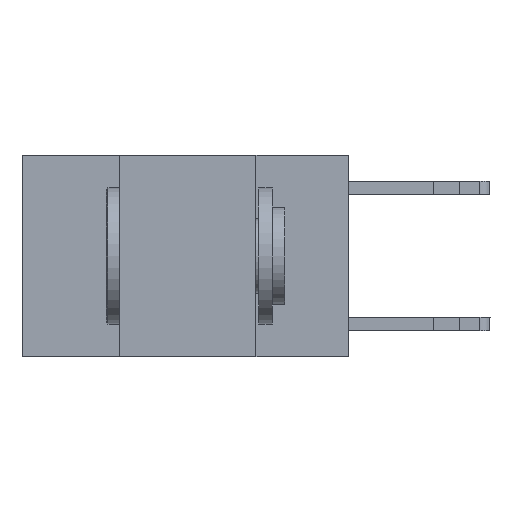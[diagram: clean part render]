
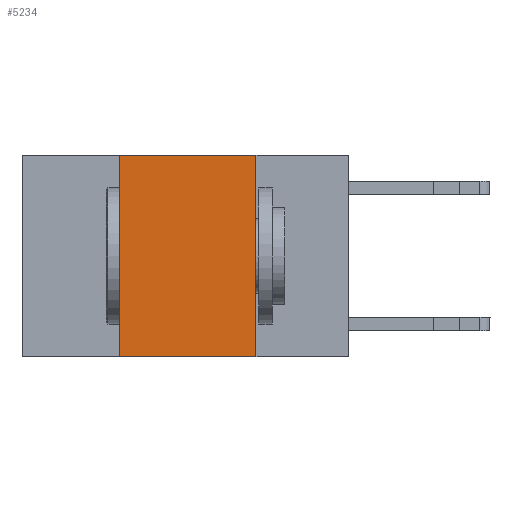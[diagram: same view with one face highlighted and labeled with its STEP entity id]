
A CAD part, left-side view. The second image highlights one B-rep face of the part: STEP entity #5234.
In plain terms, the highlighted planar face has unit normal (-1, 0, 0).
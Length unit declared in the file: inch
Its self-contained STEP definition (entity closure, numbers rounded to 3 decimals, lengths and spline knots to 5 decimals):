
#290 = EDGE_CURVE ( 'NONE', #2640, #7849, #19340, .T. ) ;
#1098 = DIRECTION ( 'NONE',  ( 0., -1., 0. ) ) ;
#1115 = EDGE_CURVE ( 'NONE', #14943, #3044, #10456, .T. ) ;
#2640 = VERTEX_POINT ( 'NONE', #4321 ) ;
#3044 = VERTEX_POINT ( 'NONE', #13803 ) ;
#3293 = EDGE_LOOP ( 'NONE', ( #13254, #5733, #10950, #13672 ) ) ;
#4226 = LINE ( 'NONE', #14617, #7386 ) ;
#4321 = CARTESIAN_POINT ( 'NONE',  ( 0., 0.42, -0.37 ) ) ;
#5234 = ADVANCED_FACE ( 'NONE', ( #9449 ), #14995, .F. ) ;
#5733 = ORIENTED_EDGE ( 'NONE', *, *, #19058, .F. ) ;
#6056 = DIRECTION ( 'NONE',  ( 1., 0., 0. ) ) ;
#7386 = VECTOR ( 'NONE', #1098, 39.37008 ) ;
#7849 = VERTEX_POINT ( 'NONE', #13498 ) ;
#7920 = DIRECTION ( 'NONE',  ( 0., -1., 0. ) ) ;
#9449 = FACE_OUTER_BOUND ( 'NONE', #3293, .T. ) ;
#10456 = LINE ( 'NONE', #13245, #17816 ) ;
#10517 = CARTESIAN_POINT ( 'NONE',  ( 0., 0.6, 0. ) ) ;
#10590 = EDGE_CURVE ( 'NONE', #2640, #3044, #4226, .T. ) ;
#10950 = ORIENTED_EDGE ( 'NONE', *, *, #290, .F. ) ;
#11636 = VECTOR ( 'NONE', #17984, 39.37008 ) ;
#12897 = DIRECTION ( 'NONE',  ( 0., 0., -1. ) ) ;
#12985 = VECTOR ( 'NONE', #7920, 39.37008 ) ;
#13014 = AXIS2_PLACEMENT_3D ( 'NONE', #10517, #6056, #16495 ) ;
#13245 = CARTESIAN_POINT ( 'NONE',  ( 0., 0.17, 0. ) ) ;
#13254 = ORIENTED_EDGE ( 'NONE', *, *, #1115, .F. ) ;
#13498 = CARTESIAN_POINT ( 'NONE',  ( 0., 0.42, 0. ) ) ;
#13672 = ORIENTED_EDGE ( 'NONE', *, *, #10590, .T. ) ;
#13803 = CARTESIAN_POINT ( 'NONE',  ( 0., 0.17, -0.37 ) ) ;
#14617 = CARTESIAN_POINT ( 'NONE',  ( 0., 0.6, -0.37 ) ) ;
#14943 = VERTEX_POINT ( 'NONE', #18679 ) ;
#14995 = PLANE ( 'NONE',  #13014 ) ;
#15978 = CARTESIAN_POINT ( 'NONE',  ( 0., 0.42, 0. ) ) ;
#16464 = LINE ( 'NONE', #16796, #12985 ) ;
#16495 = DIRECTION ( 'NONE',  ( 0., 0., -1. ) ) ;
#16796 = CARTESIAN_POINT ( 'NONE',  ( 0., 0.6, 0. ) ) ;
#17816 = VECTOR ( 'NONE', #12897, 39.37008 ) ;
#17984 = DIRECTION ( 'NONE',  ( 0., 0., 1. ) ) ;
#18679 = CARTESIAN_POINT ( 'NONE',  ( 0., 0.17, 0. ) ) ;
#19058 = EDGE_CURVE ( 'NONE', #7849, #14943, #16464, .T. ) ;
#19340 = LINE ( 'NONE', #15978, #11636 ) ;
